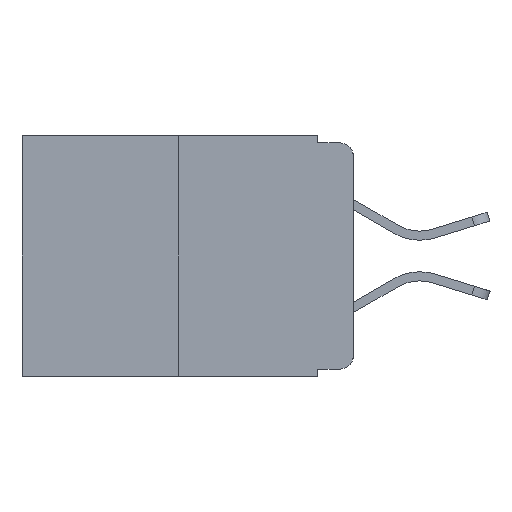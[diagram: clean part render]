
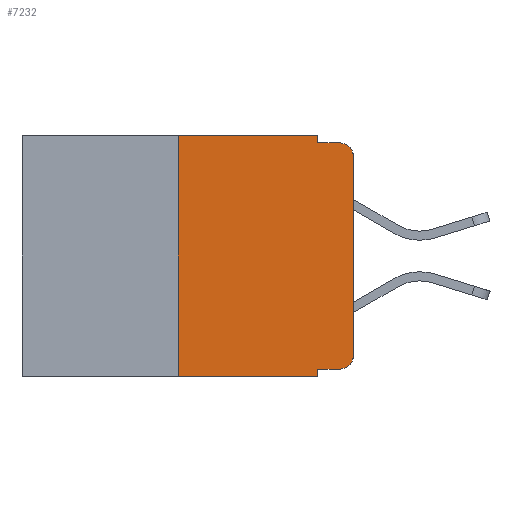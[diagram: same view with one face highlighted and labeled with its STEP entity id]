
A CAD part, left-side view. The second image highlights one B-rep face of the part: STEP entity #7232.
In plain terms, the highlighted planar face has unit normal (-1, 0, 0).
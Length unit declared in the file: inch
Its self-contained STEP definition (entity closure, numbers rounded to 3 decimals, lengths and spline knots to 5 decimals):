
#36 = DIRECTION ( 'NONE',  ( 0., 0., 1. ) ) ;
#152 = CARTESIAN_POINT ( 'NONE',  ( 0., 0.02, -0.313 ) ) ;
#215 = DIRECTION ( 'NONE',  ( 0., -1., 0. ) ) ;
#299 = EDGE_LOOP ( 'NONE', ( #8354, #9780, #8262, #12934, #2341, #9685, #4913, #10637, #7310, #3932 ) ) ;
#396 = CARTESIAN_POINT ( 'NONE',  ( 0., 0.051, -0.343 ) ) ;
#525 = LINE ( 'NONE', #11420, #3730 ) ;
#1034 = LINE ( 'NONE', #6224, #3252 ) ;
#1082 = CARTESIAN_POINT ( 'NONE',  ( 0., 0.051, 0. ) ) ;
#1467 = AXIS2_PLACEMENT_3D ( 'NONE', #152, #3128, #9114 ) ;
#1935 = CARTESIAN_POINT ( 'NONE',  ( 0., 0.051, 0. ) ) ;
#2006 = EDGE_CURVE ( 'NONE', #3353, #3890, #12066, .T. ) ;
#2154 = PLANE ( 'NONE',  #3341 ) ;
#2341 = ORIENTED_EDGE ( 'NONE', *, *, #2006, .F. ) ;
#2546 = DIRECTION ( 'NONE',  ( 0., 0., -1. ) ) ;
#2628 = DIRECTION ( 'NONE',  ( 0., -1., 0. ) ) ;
#2718 = LINE ( 'NONE', #1935, #6491 ) ;
#2910 = EDGE_CURVE ( 'NONE', #8423, #6813, #525, .T. ) ;
#2949 = VERTEX_POINT ( 'NONE', #396 ) ;
#3087 = DIRECTION ( 'NONE',  ( 0., -1., 0. ) ) ;
#3128 = DIRECTION ( 'NONE',  ( -1., 0., 0. ) ) ;
#3183 = DIRECTION ( 'NONE',  ( 0., 0., -1. ) ) ;
#3252 = VECTOR ( 'NONE', #215, 39.37008 ) ;
#3341 = AXIS2_PLACEMENT_3D ( 'NONE', #5234, #4110, #3183 ) ;
#3353 = VERTEX_POINT ( 'NONE', #3388 ) ;
#3388 = CARTESIAN_POINT ( 'NONE',  ( 0., 0.25, 0. ) ) ;
#3617 = LINE ( 'NONE', #11743, #7821 ) ;
#3730 = VECTOR ( 'NONE', #2628, 39.37008 ) ;
#3890 = VERTEX_POINT ( 'NONE', #1082 ) ;
#3932 = ORIENTED_EDGE ( 'NONE', *, *, #10804, .T. ) ;
#4110 = DIRECTION ( 'NONE',  ( 1., 0., 0. ) ) ;
#4129 = LINE ( 'NONE', #12953, #4580 ) ;
#4434 = CARTESIAN_POINT ( 'NONE',  ( 0., 0.02, -0.03 ) ) ;
#4580 = VECTOR ( 'NONE', #36, 39.37008 ) ;
#4671 = VERTEX_POINT ( 'NONE', #5508 ) ;
#4913 = ORIENTED_EDGE ( 'NONE', *, *, #12776, .T. ) ;
#5060 = EDGE_CURVE ( 'NONE', #8251, #5125, #10329, .T. ) ;
#5082 = DIRECTION ( 'NONE',  ( 0., 0., 1. ) ) ;
#5124 = CARTESIAN_POINT ( 'NONE',  ( 0., 0.473, 0. ) ) ;
#5125 = VERTEX_POINT ( 'NONE', #8521 ) ;
#5234 = CARTESIAN_POINT ( 'NONE',  ( 0., 0.473, 0. ) ) ;
#5279 = CARTESIAN_POINT ( 'NONE',  ( 0., 0., 0. ) ) ;
#5508 = CARTESIAN_POINT ( 'NONE',  ( 0., 0., -0.313 ) ) ;
#6117 = EDGE_CURVE ( 'NONE', #8423, #2949, #3617, .T. ) ;
#6128 = VERTEX_POINT ( 'NONE', #9628 ) ;
#6224 = CARTESIAN_POINT ( 'NONE',  ( 0., 0.051, -0.01 ) ) ;
#6297 = CARTESIAN_POINT ( 'NONE',  ( 0., 0.051, -0.01 ) ) ;
#6491 = VECTOR ( 'NONE', #11690, 39.37008 ) ;
#6633 = VECTOR ( 'NONE', #7763, 39.37008 ) ;
#6724 = CIRCLE ( 'NONE', #1467, 0.02 ) ;
#6813 = VERTEX_POINT ( 'NONE', #11144 ) ;
#6847 = VERTEX_POINT ( 'NONE', #6297 ) ;
#7232 = ADVANCED_FACE ( 'NONE', ( #9252 ), #2154, .F. ) ;
#7310 = ORIENTED_EDGE ( 'NONE', *, *, #2910, .T. ) ;
#7483 = EDGE_CURVE ( 'NONE', #3890, #6847, #2718, .T. ) ;
#7725 = EDGE_CURVE ( 'NONE', #4671, #8251, #10223, .T. ) ;
#7763 = DIRECTION ( 'NONE',  ( 0., -1., 0. ) ) ;
#7821 = VECTOR ( 'NONE', #12782, 39.37008 ) ;
#8251 = VERTEX_POINT ( 'NONE', #12379 ) ;
#8262 = ORIENTED_EDGE ( 'NONE', *, *, #12076, .F. ) ;
#8354 = ORIENTED_EDGE ( 'NONE', *, *, #7725, .T. ) ;
#8423 = VERTEX_POINT ( 'NONE', #8606 ) ;
#8455 = DIRECTION ( 'NONE',  ( -1., 0., 0. ) ) ;
#8521 = CARTESIAN_POINT ( 'NONE',  ( 0., 0.02, -0.01 ) ) ;
#8606 = CARTESIAN_POINT ( 'NONE',  ( 0., 0.051, -0.333 ) ) ;
#8620 = CARTESIAN_POINT ( 'NONE',  ( 0., 0.473, -0.343 ) ) ;
#8761 = LINE ( 'NONE', #8620, #6633 ) ;
#9114 = DIRECTION ( 'NONE',  ( 0., 0., -1. ) ) ;
#9252 = FACE_OUTER_BOUND ( 'NONE', #299, .T. ) ;
#9628 = CARTESIAN_POINT ( 'NONE',  ( 0., 0.25, -0.343 ) ) ;
#9685 = ORIENTED_EDGE ( 'NONE', *, *, #9818, .F. ) ;
#9780 = ORIENTED_EDGE ( 'NONE', *, *, #5060, .T. ) ;
#9818 = EDGE_CURVE ( 'NONE', #6128, #3353, #4129, .T. ) ;
#10030 = VECTOR ( 'NONE', #3087, 39.37008 ) ;
#10223 = LINE ( 'NONE', #5279, #12588 ) ;
#10329 = CIRCLE ( 'NONE', #11747, 0.02 ) ;
#10637 = ORIENTED_EDGE ( 'NONE', *, *, #6117, .F. ) ;
#10804 = EDGE_CURVE ( 'NONE', #6813, #4671, #6724, .T. ) ;
#11144 = CARTESIAN_POINT ( 'NONE',  ( 0., 0.02, -0.333 ) ) ;
#11420 = CARTESIAN_POINT ( 'NONE',  ( 0., 0.051, -0.333 ) ) ;
#11690 = DIRECTION ( 'NONE',  ( 0., 0., -1. ) ) ;
#11743 = CARTESIAN_POINT ( 'NONE',  ( 0., 0.051, 0. ) ) ;
#11747 = AXIS2_PLACEMENT_3D ( 'NONE', #4434, #8455, #2546 ) ;
#12066 = LINE ( 'NONE', #5124, #10030 ) ;
#12076 = EDGE_CURVE ( 'NONE', #6847, #5125, #1034, .T. ) ;
#12379 = CARTESIAN_POINT ( 'NONE',  ( 0., 0., -0.03 ) ) ;
#12588 = VECTOR ( 'NONE', #5082, 39.37008 ) ;
#12776 = EDGE_CURVE ( 'NONE', #6128, #2949, #8761, .T. ) ;
#12782 = DIRECTION ( 'NONE',  ( 0., 0., -1. ) ) ;
#12934 = ORIENTED_EDGE ( 'NONE', *, *, #7483, .F. ) ;
#12953 = CARTESIAN_POINT ( 'NONE',  ( 0., 0.25, 0. ) ) ;
